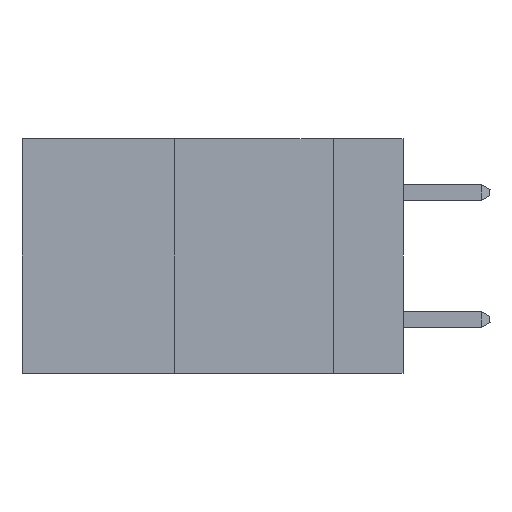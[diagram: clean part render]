
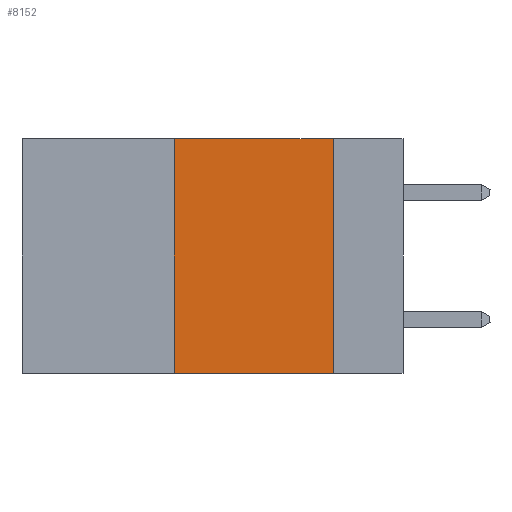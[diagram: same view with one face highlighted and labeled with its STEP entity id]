
A CAD part, left-side view. The second image highlights one B-rep face of the part: STEP entity #8152.
In plain terms, the highlighted planar face has unit normal (-1, 0, 0).
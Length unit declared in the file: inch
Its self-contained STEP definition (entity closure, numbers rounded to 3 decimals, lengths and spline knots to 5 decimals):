
#552 = VERTEX_POINT ( 'NONE', #8609 ) ;
#601 = CARTESIAN_POINT ( 'NONE',  ( 0., 0.6, 0. ) ) ;
#655 = DIRECTION ( 'NONE',  ( 0., -1., 0. ) ) ;
#831 = EDGE_CURVE ( 'NONE', #3084, #1846, #9014, .T. ) ;
#875 = DIRECTION ( 'NONE',  ( 0., -1., 0. ) ) ;
#1162 = CARTESIAN_POINT ( 'NONE',  ( 0., 0.36, 0. ) ) ;
#1846 = VERTEX_POINT ( 'NONE', #10038 ) ;
#2106 = DIRECTION ( 'NONE',  ( 0., 0., -1. ) ) ;
#2484 = VERTEX_POINT ( 'NONE', #5820 ) ;
#3084 = VERTEX_POINT ( 'NONE', #1162 ) ;
#3839 = VECTOR ( 'NONE', #655, 39.37008 ) ;
#4132 = LINE ( 'NONE', #7564, #10749 ) ;
#4710 = LINE ( 'NONE', #8218, #7067 ) ;
#4748 = ORIENTED_EDGE ( 'NONE', *, *, #9922, .F. ) ;
#5820 = CARTESIAN_POINT ( 'NONE',  ( 0., 0.11, -0.37 ) ) ;
#6380 = VECTOR ( 'NONE', #875, 39.37008 ) ;
#6924 = LINE ( 'NONE', #8047, #6380 ) ;
#7067 = VECTOR ( 'NONE', #2106, 39.37008 ) ;
#7564 = CARTESIAN_POINT ( 'NONE',  ( 0., 0.36, 0. ) ) ;
#7909 = EDGE_CURVE ( 'NONE', #552, #2484, #6924, .T. ) ;
#8047 = CARTESIAN_POINT ( 'NONE',  ( 0., 0.6, -0.37 ) ) ;
#8112 = EDGE_LOOP ( 'NONE', ( #4748, #11075, #10966, #10746 ) ) ;
#8140 = AXIS2_PLACEMENT_3D ( 'NONE', #601, #11432, #8622 ) ;
#8152 = ADVANCED_FACE ( 'NONE', ( #10744 ), #9441, .F. ) ;
#8218 = CARTESIAN_POINT ( 'NONE',  ( 0., 0.11, 0. ) ) ;
#8609 = CARTESIAN_POINT ( 'NONE',  ( 0., 0.36, -0.37 ) ) ;
#8622 = DIRECTION ( 'NONE',  ( 0., 0., -1. ) ) ;
#9014 = LINE ( 'NONE', #9497, #3839 ) ;
#9371 = DIRECTION ( 'NONE',  ( 0., 0., 1. ) ) ;
#9441 = PLANE ( 'NONE',  #8140 ) ;
#9497 = CARTESIAN_POINT ( 'NONE',  ( 0., 0.6, 0. ) ) ;
#9922 = EDGE_CURVE ( 'NONE', #1846, #2484, #4710, .T. ) ;
#10038 = CARTESIAN_POINT ( 'NONE',  ( 0., 0.11, 0. ) ) ;
#10431 = EDGE_CURVE ( 'NONE', #552, #3084, #4132, .T. ) ;
#10744 = FACE_OUTER_BOUND ( 'NONE', #8112, .T. ) ;
#10746 = ORIENTED_EDGE ( 'NONE', *, *, #7909, .T. ) ;
#10749 = VECTOR ( 'NONE', #9371, 39.37008 ) ;
#10966 = ORIENTED_EDGE ( 'NONE', *, *, #10431, .F. ) ;
#11075 = ORIENTED_EDGE ( 'NONE', *, *, #831, .F. ) ;
#11432 = DIRECTION ( 'NONE',  ( 1., 0., 0. ) ) ;
